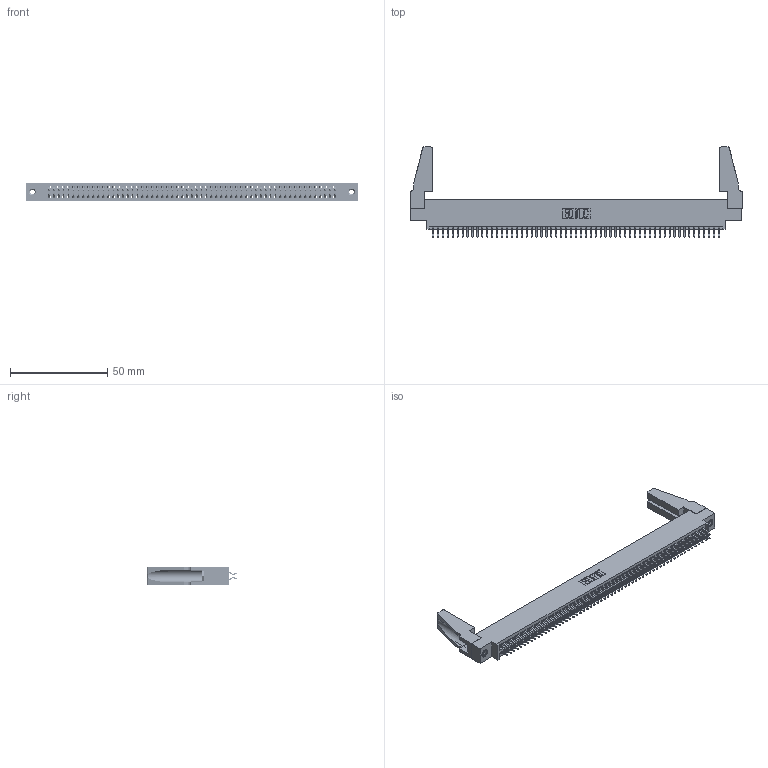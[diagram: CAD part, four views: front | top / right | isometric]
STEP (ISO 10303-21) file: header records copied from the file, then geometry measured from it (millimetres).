
FILE_DESCRIPTION (( 'STEP AP203' ), '1' );
FILE_NAME ('395-118-556-888.STEP', '2019-10-28T02:48:43', ( '' ), ( '' ), 'SwSTEP 2.0', 'SolidWorks 2016', '' );
FILE_SCHEMA (( 'CONFIG_CONTROL_DESIGN' ));
Length unit declared in the file: inch
Products named in the file (5): 345-220-078_345-220-088; 395-118-556-888; 345 Part_0.170 Offset - 0.156 Dia-TH; 345-292-001_556 Tail; 345-250-001_345-250-001-102
Assembly tree (123 placements, depth 2):
  395-118-556-888
    345 Part_0.170 Offset - 0.156 Dia-TH
    345-292-001_556 Tail  x118
    345-250-001_345-250-001-102  x2
    345-220-078_345-220-088  x2
Bounding box: 171.09 x 46.41 x 9.4 mm (x, y, z)
Volume: 19912.5 mm3; surface area: 28117.9 mm2
Topology: 123 solids, 123 shells, 6862 faces, 20373 edges, 13414 vertices
Faces by surface type: plane 4522, cylinder 2324, cone 12, torus 4
Entity records: 46504 total; most frequent: CARTESIAN_POINT 7790, ORIENTED_EDGE 7672, DIRECTION 6840, EDGE_CURVE 3836, VECTOR 3418, LINE 3418, VERTEX_POINT 2550, AXIS2_PLACEMENT_3D 1711
